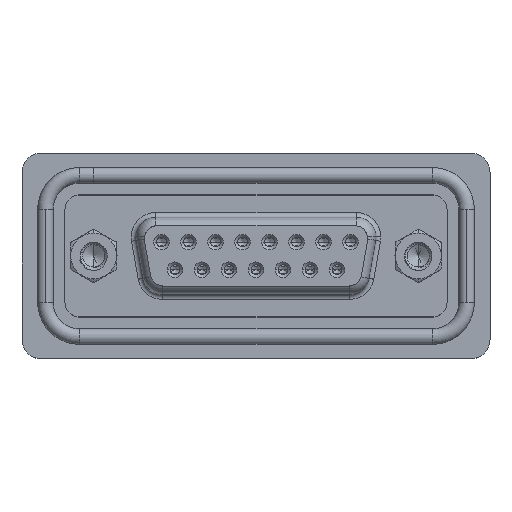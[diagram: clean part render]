
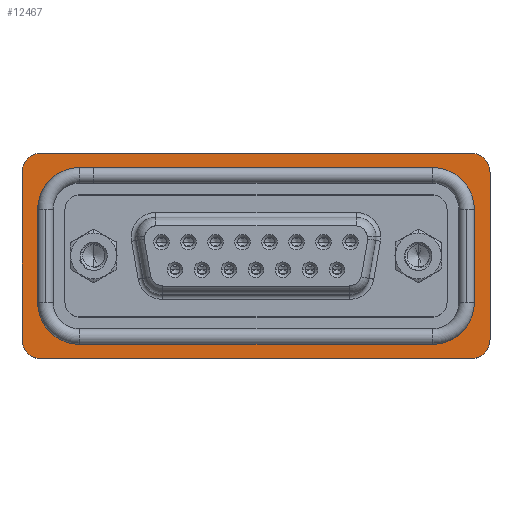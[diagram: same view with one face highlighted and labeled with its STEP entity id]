
A CAD part, top view. The second image highlights one B-rep face of the part: STEP entity #12467.
In plain terms, the highlighted planar face has unit normal (0, 0, 1).
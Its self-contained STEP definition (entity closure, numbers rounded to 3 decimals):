
#123 = DIRECTION ( 'NONE',  ( 1., 0., 0. ) ) ;
#127 = EDGE_CURVE ( 'NONE', #8991, #11242, #6550, .T. ) ;
#185 = AXIS2_PLACEMENT_3D ( 'NONE', #11524, #3647, #22722 ) ;
#375 = DIRECTION ( 'NONE',  ( 0., 0., 1. ) ) ;
#458 = DIRECTION ( 'NONE',  ( 0., 0., 1. ) ) ;
#504 = ORIENTED_EDGE ( 'NONE', *, *, #9118, .F. ) ;
#837 = ORIENTED_EDGE ( 'NONE', *, *, #23658, .T. ) ;
#842 = DIRECTION ( 'NONE',  ( 0., 0., 1. ) ) ;
#954 = AXIS2_PLACEMENT_3D ( 'NONE', #6651, #842, #13915 ) ;
#995 = CIRCLE ( 'NONE', #23017, 4.3 ) ;
#1153 = ORIENTED_EDGE ( 'NONE', *, *, #20844, .F. ) ;
#1270 = ORIENTED_EDGE ( 'NONE', *, *, #21388, .F. ) ;
#1483 = CARTESIAN_POINT ( 'NONE',  ( -5.75, -4.775, 0.5 ) ) ;
#1763 = AXIS2_PLACEMENT_3D ( 'NONE', #14090, #16172, #23668 ) ;
#1836 = VECTOR ( 'NONE', #123, 1000. ) ;
#2128 = DIRECTION ( 'NONE',  ( 0., 0., 1. ) ) ;
#2510 = LINE ( 'NONE', #21338, #5758 ) ;
#2560 = VECTOR ( 'NONE', #13387, 1000. ) ;
#3567 = VECTOR ( 'NONE', #4566, 1000. ) ;
#3647 = DIRECTION ( 'NONE',  ( 0., 0., 1. ) ) ;
#3653 = ORIENTED_EDGE ( 'NONE', *, *, #9870, .T. ) ;
#4132 = CARTESIAN_POINT ( 'NONE',  ( 40.65, -8.55, 0.5 ) ) ;
#4566 = DIRECTION ( 'NONE',  ( 0., 1., 0. ) ) ;
#5592 = VECTOR ( 'NONE', #12026, 1000. ) ;
#5624 = VERTEX_POINT ( 'NONE', #13664 ) ;
#5758 = VECTOR ( 'NONE', #7712, 1000. ) ;
#5859 = LINE ( 'NONE', #20623, #2560 ) ;
#6334 = EDGE_CURVE ( 'NONE', #7810, #15020, #8942, .T. ) ;
#6371 = DIRECTION ( 'NONE',  ( 0., -1., 0. ) ) ;
#6396 = PLANE ( 'NONE',  #954 ) ;
#6550 = LINE ( 'NONE', #15550, #3567 ) ;
#6651 = CARTESIAN_POINT ( 'NONE',  ( 38.65, 8.55, 0.5 ) ) ;
#6957 = EDGE_LOOP ( 'NONE', ( #1270, #10949, #1153, #504, #13791, #20384, #7672, #6970 ) ) ;
#6970 = ORIENTED_EDGE ( 'NONE', *, *, #6334, .F. ) ;
#7569 = CARTESIAN_POINT ( 'NONE',  ( -1.45, 9.075, 0.5 ) ) ;
#7672 = ORIENTED_EDGE ( 'NONE', *, *, #22816, .F. ) ;
#7712 = DIRECTION ( 'NONE',  ( 0., 1., 0. ) ) ;
#7713 = CARTESIAN_POINT ( 'NONE',  ( -5.75, 4.775, 0.5 ) ) ;
#7762 = ORIENTED_EDGE ( 'NONE', *, *, #127, .T. ) ;
#7810 = VERTEX_POINT ( 'NONE', #13986 ) ;
#8137 = CARTESIAN_POINT ( 'NONE',  ( -5.35, 10.55, 0.5 ) ) ;
#8942 = LINE ( 'NONE', #20000, #9513 ) ;
#8991 = VERTEX_POINT ( 'NONE', #4132 ) ;
#9118 = EDGE_CURVE ( 'NONE', #15447, #14303, #15717, .T. ) ;
#9370 = ORIENTED_EDGE ( 'NONE', *, *, #14777, .T. ) ;
#9513 = VECTOR ( 'NONE', #10416, 1000. ) ;
#9729 = VERTEX_POINT ( 'NONE', #1483 ) ;
#9814 = ORIENTED_EDGE ( 'NONE', *, *, #15072, .T. ) ;
#9870 = EDGE_CURVE ( 'NONE', #15237, #8991, #22153, .T. ) ;
#10315 = CARTESIAN_POINT ( 'NONE',  ( -5.75, 4.775, 0.5 ) ) ;
#10399 = DIRECTION ( 'NONE',  ( 1., 0., 0. ) ) ;
#10416 = DIRECTION ( 'NONE',  ( -1., 0., 0. ) ) ;
#10671 = VERTEX_POINT ( 'NONE', #21578 ) ;
#10871 = CIRCLE ( 'NONE', #23060, 2. ) ;
#10949 = ORIENTED_EDGE ( 'NONE', *, *, #23210, .F. ) ;
#11019 = CARTESIAN_POINT ( 'NONE',  ( -5.35, -8.55, 0.5 ) ) ;
#11091 = CARTESIAN_POINT ( 'NONE',  ( 38.65, -8.55, 0.5 ) ) ;
#11219 = CIRCLE ( 'NONE', #185, 2. ) ;
#11242 = VERTEX_POINT ( 'NONE', #17656 ) ;
#11250 = VECTOR ( 'NONE', #6371, 1000. ) ;
#11347 = LINE ( 'NONE', #18828, #1836 ) ;
#11449 = DIRECTION ( 'NONE',  ( 0., 0., 1. ) ) ;
#11494 = EDGE_CURVE ( 'NONE', #11242, #10671, #22989, .T. ) ;
#11524 = CARTESIAN_POINT ( 'NONE',  ( -5.35, 8.55, 0.5 ) ) ;
#11627 = DIRECTION ( 'NONE',  ( 1., 0., 0. ) ) ;
#11810 = DIRECTION ( 'NONE',  ( 1., 0., 0. ) ) ;
#11983 = DIRECTION ( 'NONE',  ( 0., -1., 0. ) ) ;
#12026 = DIRECTION ( 'NONE',  ( 1., 0., 0. ) ) ;
#12028 = EDGE_LOOP ( 'NONE', ( #23335, #21183, #16352, #9814, #9370, #837, #3653, #7762 ) ) ;
#12467 = ADVANCED_FACE ( 'NONE', ( #20041, #23379 ), #6396, .T. ) ;
#12830 = VERTEX_POINT ( 'NONE', #23589 ) ;
#12972 = CARTESIAN_POINT ( 'NONE',  ( -7.35, -8.55, 0.5 ) ) ;
#13231 = CIRCLE ( 'NONE', #17134, 4.3 ) ;
#13387 = DIRECTION ( 'NONE',  ( -1., 0., 0. ) ) ;
#13452 = CARTESIAN_POINT ( 'NONE',  ( 34.75, 4.775, 0.5 ) ) ;
#13455 = VERTEX_POINT ( 'NONE', #8137 ) ;
#13524 = AXIS2_PLACEMENT_3D ( 'NONE', #11091, #11449, #18936 ) ;
#13664 = CARTESIAN_POINT ( 'NONE',  ( 39.05, -4.775, 0.5 ) ) ;
#13740 = DIRECTION ( 'NONE',  ( 0., 0., 1. ) ) ;
#13791 = ORIENTED_EDGE ( 'NONE', *, *, #22020, .F. ) ;
#13915 = DIRECTION ( 'NONE',  ( 1., 0., 0. ) ) ;
#13955 = CARTESIAN_POINT ( 'NONE',  ( 34.75, -4.775, 0.5 ) ) ;
#13986 = CARTESIAN_POINT ( 'NONE',  ( 34.75, 9.075, 0.5 ) ) ;
#14090 = CARTESIAN_POINT ( 'NONE',  ( 38.65, 8.55, 0.5 ) ) ;
#14149 = EDGE_CURVE ( 'NONE', #24173, #9729, #20015, .T. ) ;
#14303 = VERTEX_POINT ( 'NONE', #16698 ) ;
#14436 = VECTOR ( 'NONE', #11983, 1000. ) ;
#14617 = CARTESIAN_POINT ( 'NONE',  ( 39.05, 4.775, 0.5 ) ) ;
#14777 = EDGE_CURVE ( 'NONE', #19295, #18485, #10871, .T. ) ;
#15020 = VERTEX_POINT ( 'NONE', #7569 ) ;
#15072 = EDGE_CURVE ( 'NONE', #12830, #19295, #17737, .T. ) ;
#15237 = VERTEX_POINT ( 'NONE', #23541 ) ;
#15447 = VERTEX_POINT ( 'NONE', #19519 ) ;
#15550 = CARTESIAN_POINT ( 'NONE',  ( 40.65, -8.55, 0.5 ) ) ;
#15594 = CARTESIAN_POINT ( 'NONE',  ( -1.45, -9.075, 0.5 ) ) ;
#15717 = LINE ( 'NONE', #15594, #5592 ) ;
#15984 = AXIS2_PLACEMENT_3D ( 'NONE', #19728, #13740, #10399 ) ;
#16172 = DIRECTION ( 'NONE',  ( 0., 0., 1. ) ) ;
#16352 = ORIENTED_EDGE ( 'NONE', *, *, #20242, .T. ) ;
#16698 = CARTESIAN_POINT ( 'NONE',  ( 34.75, -9.075, 0.5 ) ) ;
#17127 = DIRECTION ( 'NONE',  ( 1., 0., 0. ) ) ;
#17134 = AXIS2_PLACEMENT_3D ( 'NONE', #13452, #375, #17127 ) ;
#17656 = CARTESIAN_POINT ( 'NONE',  ( 40.65, 8.55, 0.5 ) ) ;
#17737 = LINE ( 'NONE', #19826, #14436 ) ;
#17923 = CIRCLE ( 'NONE', #15984, 4.3 ) ;
#18136 = DIRECTION ( 'NONE',  ( 0., 0., 1. ) ) ;
#18485 = VERTEX_POINT ( 'NONE', #20297 ) ;
#18828 = CARTESIAN_POINT ( 'NONE',  ( 38.65, -10.55, 0.5 ) ) ;
#18936 = DIRECTION ( 'NONE',  ( 1., 0., 0. ) ) ;
#19295 = VERTEX_POINT ( 'NONE', #12972 ) ;
#19519 = CARTESIAN_POINT ( 'NONE',  ( -1.45, -9.075, 0.5 ) ) ;
#19728 = CARTESIAN_POINT ( 'NONE',  ( -1.45, -4.775, 0.5 ) ) ;
#19826 = CARTESIAN_POINT ( 'NONE',  ( -7.35, -8.55, 0.5 ) ) ;
#20000 = CARTESIAN_POINT ( 'NONE',  ( 34.75, 9.075, 0.5 ) ) ;
#20015 = LINE ( 'NONE', #10315, #11250 ) ;
#20041 = FACE_BOUND ( 'NONE', #6957, .T. ) ;
#20242 = EDGE_CURVE ( 'NONE', #13455, #12830, #11219, .T. ) ;
#20263 = EDGE_CURVE ( 'NONE', #10671, #13455, #5859, .T. ) ;
#20297 = CARTESIAN_POINT ( 'NONE',  ( -5.35, -10.55, 0.5 ) ) ;
#20384 = ORIENTED_EDGE ( 'NONE', *, *, #14149, .F. ) ;
#20623 = CARTESIAN_POINT ( 'NONE',  ( 38.65, 10.55, 0.5 ) ) ;
#20844 = EDGE_CURVE ( 'NONE', #14303, #5624, #995, .T. ) ;
#21183 = ORIENTED_EDGE ( 'NONE', *, *, #20263, .T. ) ;
#21338 = CARTESIAN_POINT ( 'NONE',  ( 39.05, -4.775, 0.5 ) ) ;
#21388 = EDGE_CURVE ( 'NONE', #23066, #7810, #13231, .T. ) ;
#21520 = CIRCLE ( 'NONE', #23502, 4.3 ) ;
#21578 = CARTESIAN_POINT ( 'NONE',  ( 38.65, 10.55, 0.5 ) ) ;
#22020 = EDGE_CURVE ( 'NONE', #9729, #15447, #17923, .T. ) ;
#22082 = DIRECTION ( 'NONE',  ( -1., 0., 0. ) ) ;
#22153 = CIRCLE ( 'NONE', #13524, 2. ) ;
#22722 = DIRECTION ( 'NONE',  ( 1., 0., 0. ) ) ;
#22816 = EDGE_CURVE ( 'NONE', #15020, #24173, #21520, .T. ) ;
#22989 = CIRCLE ( 'NONE', #1763, 2. ) ;
#23017 = AXIS2_PLACEMENT_3D ( 'NONE', #13955, #2128, #11627 ) ;
#23060 = AXIS2_PLACEMENT_3D ( 'NONE', #11019, #18136, #22082 ) ;
#23066 = VERTEX_POINT ( 'NONE', #14617 ) ;
#23210 = EDGE_CURVE ( 'NONE', #5624, #23066, #2510, .T. ) ;
#23229 = CARTESIAN_POINT ( 'NONE',  ( -1.45, 4.775, 0.5 ) ) ;
#23335 = ORIENTED_EDGE ( 'NONE', *, *, #11494, .T. ) ;
#23379 = FACE_OUTER_BOUND ( 'NONE', #12028, .T. ) ;
#23502 = AXIS2_PLACEMENT_3D ( 'NONE', #23229, #458, #11810 ) ;
#23541 = CARTESIAN_POINT ( 'NONE',  ( 38.65, -10.55, 0.5 ) ) ;
#23589 = CARTESIAN_POINT ( 'NONE',  ( -7.35, 8.55, 0.5 ) ) ;
#23658 = EDGE_CURVE ( 'NONE', #18485, #15237, #11347, .T. ) ;
#23668 = DIRECTION ( 'NONE',  ( 1., 0., 0. ) ) ;
#24173 = VERTEX_POINT ( 'NONE', #7713 ) ;
